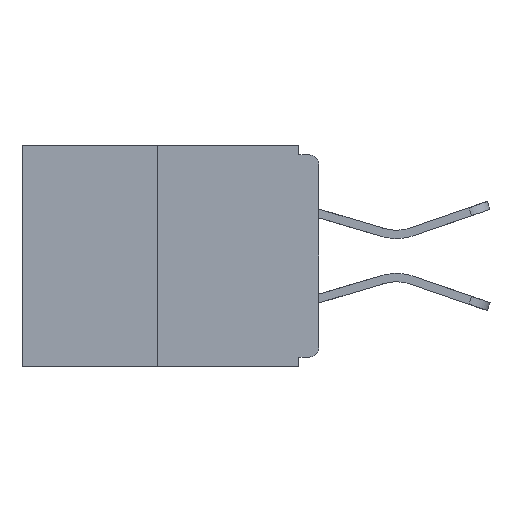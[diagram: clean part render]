
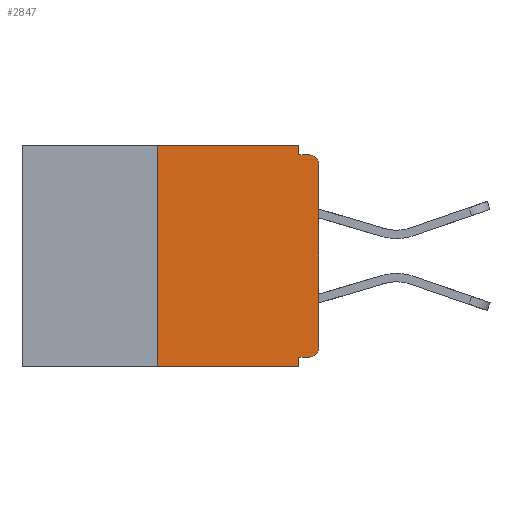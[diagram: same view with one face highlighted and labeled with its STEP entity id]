
A CAD part, left-side view. The second image highlights one B-rep face of the part: STEP entity #2847.
In plain terms, the highlighted planar face has unit normal (-1, 0, 0).
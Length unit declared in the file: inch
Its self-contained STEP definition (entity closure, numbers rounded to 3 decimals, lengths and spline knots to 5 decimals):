
#88 = EDGE_CURVE ( 'NONE', #11592, #7823, #10242, .T. ) ;
#168 = VERTEX_POINT ( 'NONE', #868 ) ;
#206 = DIRECTION ( 'NONE',  ( 0., 0., -1. ) ) ;
#228 = ORIENTED_EDGE ( 'NONE', *, *, #5599, .F. ) ;
#399 = CARTESIAN_POINT ( 'NONE',  ( 0., 0.015, -0.313 ) ) ;
#539 = VERTEX_POINT ( 'NONE', #4223 ) ;
#639 = ORIENTED_EDGE ( 'NONE', *, *, #10785, .F. ) ;
#669 = LINE ( 'NONE', #11527, #10546 ) ;
#758 = DIRECTION ( 'NONE',  ( -1., 0., 0. ) ) ;
#781 = CARTESIAN_POINT ( 'NONE',  ( 0., 0.031, 0. ) ) ;
#868 = CARTESIAN_POINT ( 'NONE',  ( 0., 0., -0.313 ) ) ;
#1263 = ORIENTED_EDGE ( 'NONE', *, *, #10362, .T. ) ;
#1403 = EDGE_CURVE ( 'NONE', #539, #6162, #13170, .T. ) ;
#1463 = LINE ( 'NONE', #2517, #3438 ) ;
#1656 = LINE ( 'NONE', #3694, #6053 ) ;
#1771 = EDGE_LOOP ( 'NONE', ( #6913, #5270, #5766, #228, #639, #2892, #2079, #1263, #3876, #3255 ) ) ;
#1969 = CARTESIAN_POINT ( 'NONE',  ( 0., 0.46, 0. ) ) ;
#2079 = ORIENTED_EDGE ( 'NONE', *, *, #8636, .T. ) ;
#2517 = CARTESIAN_POINT ( 'NONE',  ( 0., 0.46, -0.343 ) ) ;
#2847 = ADVANCED_FACE ( 'NONE', ( #7238 ), #9328, .F. ) ;
#2892 = ORIENTED_EDGE ( 'NONE', *, *, #11786, .T. ) ;
#2962 = DIRECTION ( 'NONE',  ( 0., 1., 0. ) ) ;
#3255 = ORIENTED_EDGE ( 'NONE', *, *, #8419, .F. ) ;
#3438 = VECTOR ( 'NONE', #5898, 39.37008 ) ;
#3582 = CARTESIAN_POINT ( 'NONE',  ( 0., 0., -0.03 ) ) ;
#3642 = CARTESIAN_POINT ( 'NONE',  ( 0., 0.015, -0.328 ) ) ;
#3694 = CARTESIAN_POINT ( 'NONE',  ( 0., 0., 0. ) ) ;
#3876 = ORIENTED_EDGE ( 'NONE', *, *, #1403, .F. ) ;
#4208 = DIRECTION ( 'NONE',  ( 0., 0., -1. ) ) ;
#4223 = CARTESIAN_POINT ( 'NONE',  ( 0., 0.031, -0.015 ) ) ;
#4838 = VERTEX_POINT ( 'NONE', #3582 ) ;
#4959 = DIRECTION ( 'NONE',  ( 0., 0., 1. ) ) ;
#5077 = VERTEX_POINT ( 'NONE', #11118 ) ;
#5120 = LINE ( 'NONE', #9384, #8924 ) ;
#5212 = LINE ( 'NONE', #13611, #10589 ) ;
#5270 = ORIENTED_EDGE ( 'NONE', *, *, #5702, .F. ) ;
#5599 = EDGE_CURVE ( 'NONE', #5077, #9987, #669, .T. ) ;
#5702 = EDGE_CURVE ( 'NONE', #10588, #11592, #9362, .T. ) ;
#5766 = ORIENTED_EDGE ( 'NONE', *, *, #9794, .T. ) ;
#5898 = DIRECTION ( 'NONE',  ( 0., -1., 0. ) ) ;
#5929 = VECTOR ( 'NONE', #13376, 39.37008 ) ;
#6053 = VECTOR ( 'NONE', #7901, 39.37008 ) ;
#6148 = AXIS2_PLACEMENT_3D ( 'NONE', #399, #6618, #206 ) ;
#6162 = VERTEX_POINT ( 'NONE', #12475 ) ;
#6266 = DIRECTION ( 'NONE',  ( 1., 0., 0. ) ) ;
#6618 = DIRECTION ( 'NONE',  ( -1., 0., 0. ) ) ;
#6635 = VECTOR ( 'NONE', #10098, 39.37008 ) ;
#6838 = CARTESIAN_POINT ( 'NONE',  ( 0., 0.46, 0. ) ) ;
#6913 = ORIENTED_EDGE ( 'NONE', *, *, #88, .F. ) ;
#7238 = FACE_OUTER_BOUND ( 'NONE', #1771, .T. ) ;
#7678 = CIRCLE ( 'NONE', #11232, 0.015 ) ;
#7823 = VERTEX_POINT ( 'NONE', #781 ) ;
#7901 = DIRECTION ( 'NONE',  ( 0., 0., 1. ) ) ;
#8114 = AXIS2_PLACEMENT_3D ( 'NONE', #1969, #6266, #13602 ) ;
#8178 = CARTESIAN_POINT ( 'NONE',  ( 0., 0.25, 0. ) ) ;
#8179 = VERTEX_POINT ( 'NONE', #3642 ) ;
#8419 = EDGE_CURVE ( 'NONE', #7823, #539, #5120, .T. ) ;
#8636 = EDGE_CURVE ( 'NONE', #168, #4838, #1656, .T. ) ;
#8924 = VECTOR ( 'NONE', #4208, 39.37008 ) ;
#9328 = PLANE ( 'NONE',  #8114 ) ;
#9362 = LINE ( 'NONE', #8178, #9874 ) ;
#9384 = CARTESIAN_POINT ( 'NONE',  ( 0., 0.031, 0. ) ) ;
#9794 = EDGE_CURVE ( 'NONE', #10588, #9987, #1463, .T. ) ;
#9874 = VECTOR ( 'NONE', #4959, 39.37008 ) ;
#9924 = CIRCLE ( 'NONE', #6148, 0.015 ) ;
#9987 = VERTEX_POINT ( 'NONE', #13527 ) ;
#10098 = DIRECTION ( 'NONE',  ( 0., -1., 0. ) ) ;
#10242 = LINE ( 'NONE', #6838, #6635 ) ;
#10362 = EDGE_CURVE ( 'NONE', #4838, #6162, #7678, .T. ) ;
#10475 = DIRECTION ( 'NONE',  ( 0., 0., -1. ) ) ;
#10546 = VECTOR ( 'NONE', #10475, 39.37008 ) ;
#10588 = VERTEX_POINT ( 'NONE', #11446 ) ;
#10589 = VECTOR ( 'NONE', #2962, 39.37008 ) ;
#10785 = EDGE_CURVE ( 'NONE', #8179, #5077, #5212, .T. ) ;
#11080 = CARTESIAN_POINT ( 'NONE',  ( 0., 0.25, 0. ) ) ;
#11118 = CARTESIAN_POINT ( 'NONE',  ( 0., 0.031, -0.328 ) ) ;
#11232 = AXIS2_PLACEMENT_3D ( 'NONE', #12435, #758, #13649 ) ;
#11446 = CARTESIAN_POINT ( 'NONE',  ( 0., 0.25, -0.343 ) ) ;
#11527 = CARTESIAN_POINT ( 'NONE',  ( 0., 0.031, -0.343 ) ) ;
#11592 = VERTEX_POINT ( 'NONE', #11080 ) ;
#11786 = EDGE_CURVE ( 'NONE', #8179, #168, #9924, .T. ) ;
#12104 = CARTESIAN_POINT ( 'NONE',  ( 0., 0., -0.015 ) ) ;
#12435 = CARTESIAN_POINT ( 'NONE',  ( 0., 0.015, -0.03 ) ) ;
#12475 = CARTESIAN_POINT ( 'NONE',  ( 0., 0.015, -0.015 ) ) ;
#13170 = LINE ( 'NONE', #12104, #5929 ) ;
#13376 = DIRECTION ( 'NONE',  ( 0., -1., 0. ) ) ;
#13527 = CARTESIAN_POINT ( 'NONE',  ( 0., 0.031, -0.343 ) ) ;
#13602 = DIRECTION ( 'NONE',  ( 0., 0., -1. ) ) ;
#13611 = CARTESIAN_POINT ( 'NONE',  ( 0., 0., -0.328 ) ) ;
#13649 = DIRECTION ( 'NONE',  ( 0., 0., -1. ) ) ;
